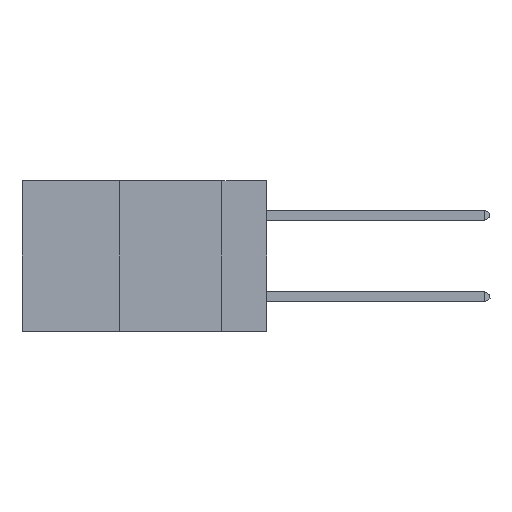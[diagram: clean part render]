
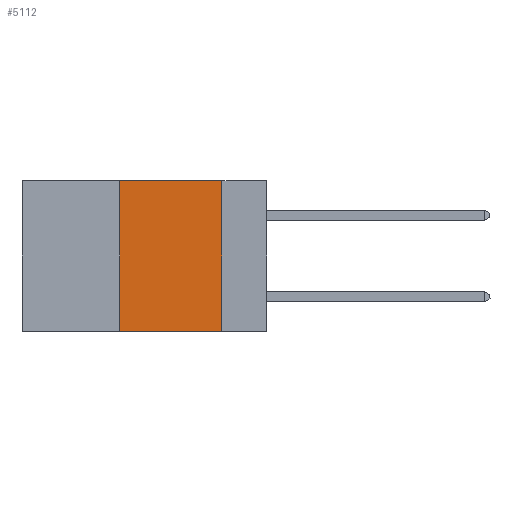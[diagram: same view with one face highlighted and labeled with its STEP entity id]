
A CAD part, left-side view. The second image highlights one B-rep face of the part: STEP entity #5112.
In plain terms, the highlighted planar face has unit normal (-1, 0, 0).
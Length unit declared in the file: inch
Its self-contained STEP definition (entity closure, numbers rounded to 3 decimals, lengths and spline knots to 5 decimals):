
#322 = DIRECTION ( 'NONE',  ( 0., -1., 0. ) ) ;
#399 = VERTEX_POINT ( 'NONE', #2942 ) ;
#625 = VERTEX_POINT ( 'NONE', #9009 ) ;
#780 = CARTESIAN_POINT ( 'NONE',  ( 0., 0.36, 0. ) ) ;
#788 = FACE_OUTER_BOUND ( 'NONE', #5298, .T. ) ;
#1169 = PLANE ( 'NONE',  #8766 ) ;
#1261 = CARTESIAN_POINT ( 'NONE',  ( 0., 0.11, 0. ) ) ;
#1412 = CARTESIAN_POINT ( 'NONE',  ( 0., 0.36, -0.37 ) ) ;
#1667 = DIRECTION ( 'NONE',  ( 0., 0., -1. ) ) ;
#2330 = DIRECTION ( 'NONE',  ( 0., 0., 1. ) ) ;
#2718 = CARTESIAN_POINT ( 'NONE',  ( 0., 0.6, 0. ) ) ;
#2942 = CARTESIAN_POINT ( 'NONE',  ( 0., 0.36, 0. ) ) ;
#3091 = ORIENTED_EDGE ( 'NONE', *, *, #6767, .F. ) ;
#3827 = EDGE_CURVE ( 'NONE', #399, #8457, #8063, .T. ) ;
#4475 = EDGE_CURVE ( 'NONE', #6090, #625, #9369, .T. ) ;
#4545 = DIRECTION ( 'NONE',  ( 1., 0., 0. ) ) ;
#4569 = DIRECTION ( 'NONE',  ( 0., -1., 0. ) ) ;
#4724 = ORIENTED_EDGE ( 'NONE', *, *, #9307, .F. ) ;
#4971 = DIRECTION ( 'NONE',  ( 0., 0., -1. ) ) ;
#5112 = ADVANCED_FACE ( 'NONE', ( #788 ), #1169, .F. ) ;
#5188 = VECTOR ( 'NONE', #4971, 39.37008 ) ;
#5298 = EDGE_LOOP ( 'NONE', ( #3091, #9455, #4724, #6359 ) ) ;
#5610 = LINE ( 'NONE', #780, #7850 ) ;
#5697 = CARTESIAN_POINT ( 'NONE',  ( 0., 0.11, 0. ) ) ;
#6047 = VECTOR ( 'NONE', #4569, 39.37008 ) ;
#6059 = CARTESIAN_POINT ( 'NONE',  ( 0., 0.6, -0.37 ) ) ;
#6090 = VERTEX_POINT ( 'NONE', #1412 ) ;
#6359 = ORIENTED_EDGE ( 'NONE', *, *, #4475, .T. ) ;
#6767 = EDGE_CURVE ( 'NONE', #8457, #625, #7762, .T. ) ;
#7217 = VECTOR ( 'NONE', #322, 39.37008 ) ;
#7762 = LINE ( 'NONE', #1261, #5188 ) ;
#7850 = VECTOR ( 'NONE', #2330, 39.37008 ) ;
#8063 = LINE ( 'NONE', #8510, #7217 ) ;
#8457 = VERTEX_POINT ( 'NONE', #5697 ) ;
#8510 = CARTESIAN_POINT ( 'NONE',  ( 0., 0.6, 0. ) ) ;
#8766 = AXIS2_PLACEMENT_3D ( 'NONE', #2718, #4545, #1667 ) ;
#9009 = CARTESIAN_POINT ( 'NONE',  ( 0., 0.11, -0.37 ) ) ;
#9307 = EDGE_CURVE ( 'NONE', #6090, #399, #5610, .T. ) ;
#9369 = LINE ( 'NONE', #6059, #6047 ) ;
#9455 = ORIENTED_EDGE ( 'NONE', *, *, #3827, .F. ) ;
